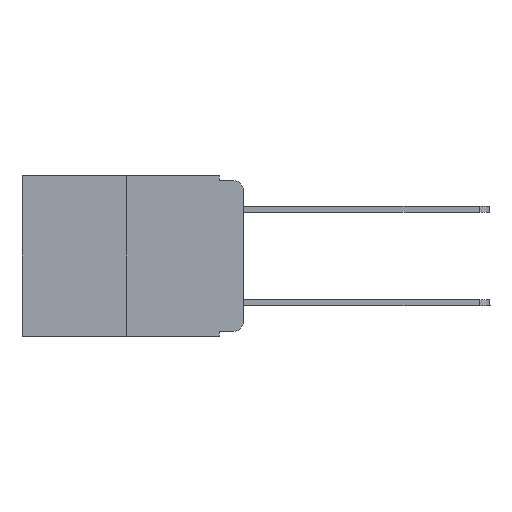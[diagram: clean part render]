
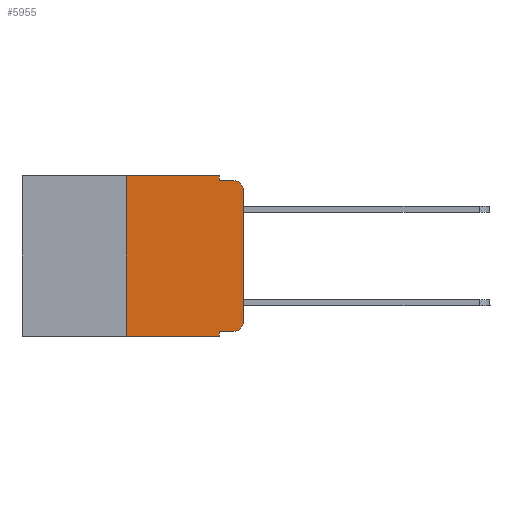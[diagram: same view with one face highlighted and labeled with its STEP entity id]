
A CAD part, left-side view. The second image highlights one B-rep face of the part: STEP entity #5955.
In plain terms, the highlighted planar face has unit normal (-1, 0, 0).
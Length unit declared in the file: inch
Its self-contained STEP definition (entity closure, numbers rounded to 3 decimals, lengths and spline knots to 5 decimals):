
#393 = VECTOR ( 'NONE', #13246, 39.37008 ) ;
#599 = VERTEX_POINT ( 'NONE', #15778 ) ;
#695 = CARTESIAN_POINT ( 'NONE',  ( 0., 0.02, -0.01 ) ) ;
#752 = DIRECTION ( 'NONE',  ( 0., 0., -1. ) ) ;
#863 = ORIENTED_EDGE ( 'NONE', *, *, #9292, .F. ) ;
#982 = DIRECTION ( 'NONE',  ( 0., -1., 0. ) ) ;
#985 = CARTESIAN_POINT ( 'NONE',  ( 0., 0.051, 0. ) ) ;
#1316 = CARTESIAN_POINT ( 'NONE',  ( 0., 0.25, 0. ) ) ;
#1318 = CARTESIAN_POINT ( 'NONE',  ( 0., 0., -0.313 ) ) ;
#1488 = EDGE_CURVE ( 'NONE', #6556, #1735, #17999, .T. ) ;
#1543 = ORIENTED_EDGE ( 'NONE', *, *, #17387, .T. ) ;
#1592 = DIRECTION ( 'NONE',  ( 0., -1., 0. ) ) ;
#1735 = VERTEX_POINT ( 'NONE', #695 ) ;
#1757 = ORIENTED_EDGE ( 'NONE', *, *, #16276, .T. ) ;
#1918 = DIRECTION ( 'NONE',  ( -1., 0., 0. ) ) ;
#2082 = CARTESIAN_POINT ( 'NONE',  ( 0., 0.051, -0.01 ) ) ;
#2137 = DIRECTION ( 'NONE',  ( 1., 0., 0. ) ) ;
#2265 = VECTOR ( 'NONE', #1592, 39.37008 ) ;
#2313 = LINE ( 'NONE', #16378, #6110 ) ;
#2597 = CARTESIAN_POINT ( 'NONE',  ( 0., 0.473, 0. ) ) ;
#3084 = VECTOR ( 'NONE', #4154, 39.37008 ) ;
#4000 = EDGE_LOOP ( 'NONE', ( #9336, #1757, #6857, #863, #14407, #10646, #1543, #22425, #11282, #14342 ) ) ;
#4154 = DIRECTION ( 'NONE',  ( 0., -1., 0. ) ) ;
#4157 = LINE ( 'NONE', #17403, #2265 ) ;
#4482 = EDGE_CURVE ( 'NONE', #5975, #12233, #18618, .T. ) ;
#5029 = EDGE_CURVE ( 'NONE', #12233, #19054, #2313, .T. ) ;
#5150 = DIRECTION ( 'NONE',  ( 0., 0., -1. ) ) ;
#5158 = EDGE_CURVE ( 'NONE', #11098, #14824, #13611, .T. ) ;
#5519 = CARTESIAN_POINT ( 'NONE',  ( 0., 0.051, -0.343 ) ) ;
#5751 = VECTOR ( 'NONE', #10158, 39.37008 ) ;
#5946 = FACE_OUTER_BOUND ( 'NONE', #4000, .T. ) ;
#5955 = ADVANCED_FACE ( 'NONE', ( #5946 ), #16206, .F. ) ;
#5975 = VERTEX_POINT ( 'NONE', #10920 ) ;
#6110 = VECTOR ( 'NONE', #18458, 39.37008 ) ;
#6284 = CARTESIAN_POINT ( 'NONE',  ( 0., 0.473, 0. ) ) ;
#6556 = VERTEX_POINT ( 'NONE', #13531 ) ;
#6857 = ORIENTED_EDGE ( 'NONE', *, *, #1488, .F. ) ;
#7371 = CIRCLE ( 'NONE', #12163, 0.02 ) ;
#8615 = CARTESIAN_POINT ( 'NONE',  ( 0., 0.051, 0. ) ) ;
#9292 = EDGE_CURVE ( 'NONE', #15061, #6556, #20135, .T. ) ;
#9336 = ORIENTED_EDGE ( 'NONE', *, *, #5029, .T. ) ;
#9443 = EDGE_CURVE ( 'NONE', #10818, #599, #17457, .T. ) ;
#10158 = DIRECTION ( 'NONE',  ( 0., 0., -1. ) ) ;
#10339 = CARTESIAN_POINT ( 'NONE',  ( 0., 0.02, -0.313 ) ) ;
#10571 = DIRECTION ( 'NONE',  ( 0., 0., -1. ) ) ;
#10646 = ORIENTED_EDGE ( 'NONE', *, *, #9443, .F. ) ;
#10818 = VERTEX_POINT ( 'NONE', #15504 ) ;
#10920 = CARTESIAN_POINT ( 'NONE',  ( 0., 0.02, -0.333 ) ) ;
#11098 = VERTEX_POINT ( 'NONE', #18276 ) ;
#11282 = ORIENTED_EDGE ( 'NONE', *, *, #16517, .T. ) ;
#12163 = AXIS2_PLACEMENT_3D ( 'NONE', #12547, #1918, #5150 ) ;
#12233 = VERTEX_POINT ( 'NONE', #1318 ) ;
#12547 = CARTESIAN_POINT ( 'NONE',  ( 0., 0.02, -0.03 ) ) ;
#13246 = DIRECTION ( 'NONE',  ( 0., -1., 0. ) ) ;
#13531 = CARTESIAN_POINT ( 'NONE',  ( 0., 0.051, -0.01 ) ) ;
#13611 = LINE ( 'NONE', #13719, #5751 ) ;
#13719 = CARTESIAN_POINT ( 'NONE',  ( 0., 0.051, 0. ) ) ;
#14342 = ORIENTED_EDGE ( 'NONE', *, *, #4482, .T. ) ;
#14407 = ORIENTED_EDGE ( 'NONE', *, *, #17044, .F. ) ;
#14422 = VECTOR ( 'NONE', #982, 39.37008 ) ;
#14824 = VERTEX_POINT ( 'NONE', #5519 ) ;
#15061 = VERTEX_POINT ( 'NONE', #8615 ) ;
#15504 = CARTESIAN_POINT ( 'NONE',  ( 0., 0.25, -0.343 ) ) ;
#15778 = CARTESIAN_POINT ( 'NONE',  ( 0., 0.25, 0. ) ) ;
#15862 = VECTOR ( 'NONE', #19092, 39.37008 ) ;
#16206 = PLANE ( 'NONE',  #17188 ) ;
#16276 = EDGE_CURVE ( 'NONE', #19054, #1735, #7371, .T. ) ;
#16378 = CARTESIAN_POINT ( 'NONE',  ( 0., 0., 0. ) ) ;
#16517 = EDGE_CURVE ( 'NONE', #11098, #5975, #16695, .T. ) ;
#16695 = LINE ( 'NONE', #21986, #393 ) ;
#17044 = EDGE_CURVE ( 'NONE', #599, #15061, #17544, .T. ) ;
#17138 = AXIS2_PLACEMENT_3D ( 'NONE', #10339, #19559, #10571 ) ;
#17188 = AXIS2_PLACEMENT_3D ( 'NONE', #2597, #2137, #18058 ) ;
#17387 = EDGE_CURVE ( 'NONE', #10818, #14824, #4157, .T. ) ;
#17403 = CARTESIAN_POINT ( 'NONE',  ( 0., 0.473, -0.343 ) ) ;
#17457 = LINE ( 'NONE', #1316, #15862 ) ;
#17544 = LINE ( 'NONE', #6284, #14422 ) ;
#17999 = LINE ( 'NONE', #2082, #3084 ) ;
#18058 = DIRECTION ( 'NONE',  ( 0., 0., -1. ) ) ;
#18276 = CARTESIAN_POINT ( 'NONE',  ( 0., 0.051, -0.333 ) ) ;
#18458 = DIRECTION ( 'NONE',  ( 0., 0., 1. ) ) ;
#18618 = CIRCLE ( 'NONE', #17138, 0.02 ) ;
#19054 = VERTEX_POINT ( 'NONE', #21994 ) ;
#19092 = DIRECTION ( 'NONE',  ( 0., 0., 1. ) ) ;
#19559 = DIRECTION ( 'NONE',  ( -1., 0., 0. ) ) ;
#20135 = LINE ( 'NONE', #985, #21370 ) ;
#21370 = VECTOR ( 'NONE', #752, 39.37008 ) ;
#21986 = CARTESIAN_POINT ( 'NONE',  ( 0., 0.051, -0.333 ) ) ;
#21994 = CARTESIAN_POINT ( 'NONE',  ( 0., 0., -0.03 ) ) ;
#22425 = ORIENTED_EDGE ( 'NONE', *, *, #5158, .F. ) ;
